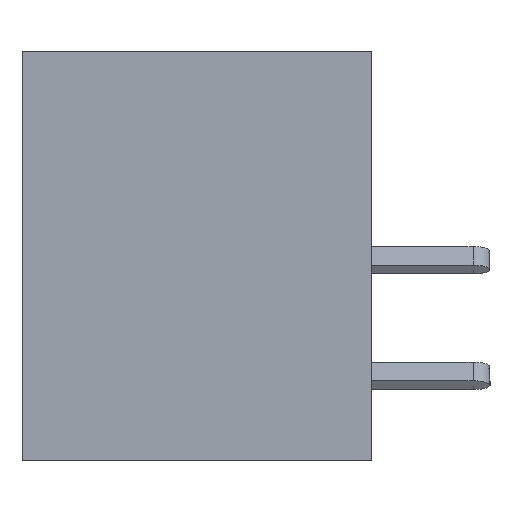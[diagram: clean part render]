
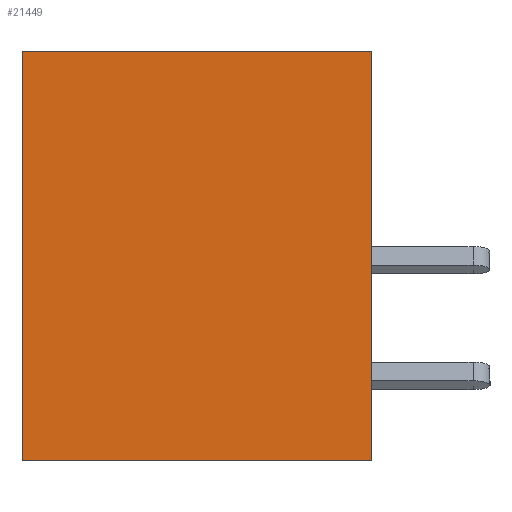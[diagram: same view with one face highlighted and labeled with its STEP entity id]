
A CAD part, left-side view. The second image highlights one B-rep face of the part: STEP entity #21449.
In plain terms, the highlighted planar face has unit normal (-1, 0, 0).
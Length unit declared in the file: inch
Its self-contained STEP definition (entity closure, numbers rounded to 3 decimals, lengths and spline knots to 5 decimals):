
#20 = DIRECTION ( 'NONE',  ( 0., 0., 1. ) ) ;
#3417 = ORIENTED_EDGE ( 'NONE', *, *, #19570, .F. ) ;
#4478 = EDGE_CURVE ( 'NONE', #27985, #16830, #9712, .T. ) ;
#5309 = CARTESIAN_POINT ( 'NONE',  ( 0., 0.453, -0.531 ) ) ;
#5564 = VECTOR ( 'NONE', #11542, 39.37008 ) ;
#5737 = VERTEX_POINT ( 'NONE', #23061 ) ;
#7180 = PLANE ( 'NONE',  #25340 ) ;
#8174 = EDGE_CURVE ( 'NONE', #5737, #27985, #28486, .T. ) ;
#8341 = VECTOR ( 'NONE', #9733, 39.37008 ) ;
#8571 = EDGE_LOOP ( 'NONE', ( #24101, #3417, #19593, #10735 ) ) ;
#9694 = EDGE_CURVE ( 'NONE', #5737, #24743, #17287, .T. ) ;
#9712 = LINE ( 'NONE', #26677, #5564 ) ;
#9733 = DIRECTION ( 'NONE',  ( 0., -1., 0. ) ) ;
#10735 = ORIENTED_EDGE ( 'NONE', *, *, #8174, .T. ) ;
#11415 = VECTOR ( 'NONE', #20, 39.37008 ) ;
#11542 = DIRECTION ( 'NONE',  ( 0., 0., 1. ) ) ;
#15927 = CARTESIAN_POINT ( 'NONE',  ( 0., 0., -0.531 ) ) ;
#16830 = VERTEX_POINT ( 'NONE', #21929 ) ;
#17287 = LINE ( 'NONE', #17699, #11415 ) ;
#17435 = VECTOR ( 'NONE', #26022, 39.37008 ) ;
#17699 = CARTESIAN_POINT ( 'NONE',  ( 0., 0.453, 0. ) ) ;
#18069 = CARTESIAN_POINT ( 'NONE',  ( 0., 0.453, 0. ) ) ;
#18346 = CARTESIAN_POINT ( 'NONE',  ( 0., 0.453, 0. ) ) ;
#19166 = CARTESIAN_POINT ( 'NONE',  ( 0., 0.453, 0. ) ) ;
#19570 = EDGE_CURVE ( 'NONE', #24743, #16830, #23357, .T. ) ;
#19593 = ORIENTED_EDGE ( 'NONE', *, *, #9694, .F. ) ;
#20571 = DIRECTION ( 'NONE',  ( 1., 0., 0. ) ) ;
#21449 = ADVANCED_FACE ( 'NONE', ( #21495 ), #7180, .F. ) ;
#21495 = FACE_OUTER_BOUND ( 'NONE', #8571, .T. ) ;
#21929 = CARTESIAN_POINT ( 'NONE',  ( 0., 0., 0. ) ) ;
#23061 = CARTESIAN_POINT ( 'NONE',  ( 0., 0.453, -0.531 ) ) ;
#23185 = DIRECTION ( 'NONE',  ( 0., 0., -1. ) ) ;
#23357 = LINE ( 'NONE', #19166, #17435 ) ;
#24101 = ORIENTED_EDGE ( 'NONE', *, *, #4478, .T. ) ;
#24743 = VERTEX_POINT ( 'NONE', #18069 ) ;
#25340 = AXIS2_PLACEMENT_3D ( 'NONE', #18346, #20571, #23185 ) ;
#26022 = DIRECTION ( 'NONE',  ( 0., -1., 0. ) ) ;
#26677 = CARTESIAN_POINT ( 'NONE',  ( 0., 0., 0. ) ) ;
#27985 = VERTEX_POINT ( 'NONE', #15927 ) ;
#28486 = LINE ( 'NONE', #5309, #8341 ) ;
